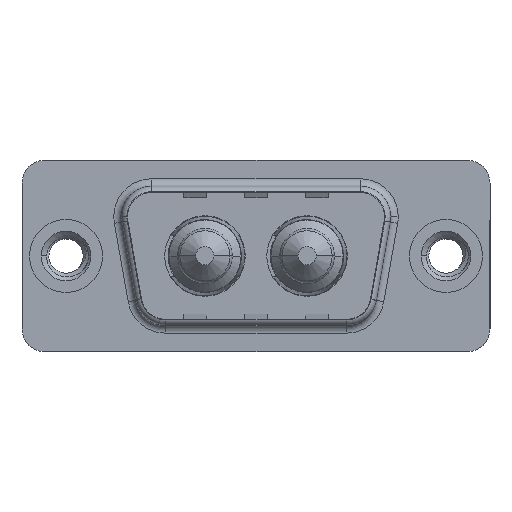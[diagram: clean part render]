
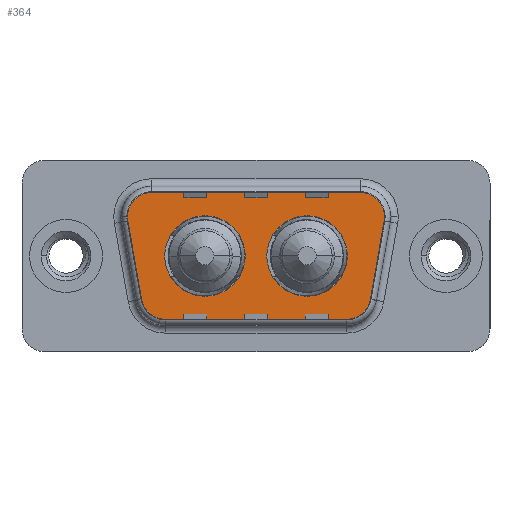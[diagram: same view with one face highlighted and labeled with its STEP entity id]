
A CAD part, top view. The second image highlights one B-rep face of the part: STEP entity #364.
In plain terms, the highlighted planar face has unit normal (0, 0, 1).
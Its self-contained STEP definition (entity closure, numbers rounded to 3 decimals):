
#38 = AXIS2_PLACEMENT_3D ( 'NONE', #1560, #8063, #2485 ) ;
#93 = CARTESIAN_POINT ( 'NONE',  ( 19.564, 2.9, 0. ) ) ;
#279 = CIRCLE ( 'NONE', #2999, 2.65 ) ;
#339 = ORIENTED_EDGE ( 'NONE', *, *, #10222, .T. ) ;
#352 = AXIS2_PLACEMENT_3D ( 'NONE', #7111, #1551, #8054 ) ;
#364 = ADVANCED_FACE ( 'NONE', ( #7872, #2904, #735 ), #11195, .T. ) ;
#393 = DIRECTION ( 'NONE',  ( 0., 0., 1. ) ) ;
#396 = AXIS2_PLACEMENT_3D ( 'NONE', #7587, #2021, #8519 ) ;
#509 = CARTESIAN_POINT ( 'NONE',  ( 15.86, 0., 0. ) ) ;
#714 = CIRCLE ( 'NONE', #3852, 2.65 ) ;
#735 = FACE_OUTER_BOUND ( 'NONE', #986, .T. ) ;
#771 = DIRECTION ( 'NONE',  ( 1., 0., 0. ) ) ;
#777 = CARTESIAN_POINT ( 'NONE',  ( 11.79, 0., 0. ) ) ;
#908 = VERTEX_POINT ( 'NONE', #11458 ) ;
#986 = EDGE_LOOP ( 'NONE', ( #3977, #2507, #9178, #2822, #2939, #3362, #339, #5074, #2088 ) ) ;
#1273 = ORIENTED_EDGE ( 'NONE', *, *, #1578, .F. ) ;
#1403 = DIRECTION ( 'NONE',  ( 1., 0., 0. ) ) ;
#1448 = DIRECTION ( 'NONE',  ( 1., 0., 0. ) ) ;
#1551 = DIRECTION ( 'NONE',  ( 0., 0., 1. ) ) ;
#1560 = CARTESIAN_POINT ( 'NONE',  ( 5.436, 2.9, 0. ) ) ;
#1578 = EDGE_CURVE ( 'NONE', #11926, #2468, #714, .T. ) ;
#1616 = CARTESIAN_POINT ( 'NONE',  ( 20.511, -3.247, 0. ) ) ;
#1685 = DIRECTION ( 'NONE',  ( -1., 0., 0. ) ) ;
#1710 = DIRECTION ( 'NONE',  ( 0., 0., 1. ) ) ;
#1712 = CARTESIAN_POINT ( 'NONE',  ( 21.564, 2.9, 0. ) ) ;
#1871 = EDGE_CURVE ( 'NONE', #2468, #11926, #279, .T. ) ;
#1943 = AXIS2_PLACEMENT_3D ( 'NONE', #509, #7012, #1448 ) ;
#1998 = CIRCLE ( 'NONE', #1943, 2.65 ) ;
#2021 = DIRECTION ( 'NONE',  ( 0., 0., 1. ) ) ;
#2088 = ORIENTED_EDGE ( 'NONE', *, *, #9169, .T. ) ;
#2161 = LINE ( 'NONE', #9250, #4331 ) ;
#2251 = VECTOR ( 'NONE', #11970, 1000. ) ;
#2264 = ORIENTED_EDGE ( 'NONE', *, *, #7090, .F. ) ;
#2468 = VERTEX_POINT ( 'NONE', #9213 ) ;
#2485 = DIRECTION ( 'NONE',  ( 1., 0., 0. ) ) ;
#2507 = ORIENTED_EDGE ( 'NONE', *, *, #4320, .T. ) ;
#2779 = EDGE_LOOP ( 'NONE', ( #2264, #5997 ) ) ;
#2822 = ORIENTED_EDGE ( 'NONE', *, *, #5196, .T. ) ;
#2904 = FACE_BOUND ( 'NONE', #9049, .T. ) ;
#2939 = ORIENTED_EDGE ( 'NONE', *, *, #6169, .T. ) ;
#2999 = AXIS2_PLACEMENT_3D ( 'NONE', #10665, #8301, #1403 ) ;
#3227 = VERTEX_POINT ( 'NONE', #1712 ) ;
#3351 = CARTESIAN_POINT ( 'NONE',  ( 18.541, -2.9, 0. ) ) ;
#3362 = ORIENTED_EDGE ( 'NONE', *, *, #9053, .T. ) ;
#3473 = EDGE_CURVE ( 'NONE', #9701, #10639, #11126, .T. ) ;
#3543 = CIRCLE ( 'NONE', #38, 2. ) ;
#3703 = CIRCLE ( 'NONE', #396, 2. ) ;
#3784 = CARTESIAN_POINT ( 'NONE',  ( 18.541, -4.9, 0. ) ) ;
#3852 = AXIS2_PLACEMENT_3D ( 'NONE', #6320, #8815, #3908 ) ;
#3908 = DIRECTION ( 'NONE',  ( 1., 0., 0. ) ) ;
#3977 = ORIENTED_EDGE ( 'NONE', *, *, #8643, .T. ) ;
#4039 = DIRECTION ( 'NONE',  ( 1., 0., 0. ) ) ;
#4287 = VECTOR ( 'NONE', #771, 1000. ) ;
#4320 = EDGE_CURVE ( 'NONE', #4610, #6914, #2161, .T. ) ;
#4331 = VECTOR ( 'NONE', #8537, 1000. ) ;
#4422 = AXIS2_PLACEMENT_3D ( 'NONE', #5977, #393, #6894 ) ;
#4610 = VERTEX_POINT ( 'NONE', #1616 ) ;
#4792 = CIRCLE ( 'NONE', #4422, 2.65 ) ;
#5074 = ORIENTED_EDGE ( 'NONE', *, *, #3473, .T. ) ;
#5196 = EDGE_CURVE ( 'NONE', #3227, #908, #9450, .T. ) ;
#5315 = LINE ( 'NONE', #11024, #2251 ) ;
#5463 = CARTESIAN_POINT ( 'NONE',  ( 5.436, 4.9, 0. ) ) ;
#5670 = VECTOR ( 'NONE', #12051, 1000. ) ;
#5899 = DIRECTION ( 'NONE',  ( 0., 0., 1. ) ) ;
#5977 = CARTESIAN_POINT ( 'NONE',  ( 15.86, 0., 0. ) ) ;
#5997 = ORIENTED_EDGE ( 'NONE', *, *, #8282, .F. ) ;
#6048 = CARTESIAN_POINT ( 'NONE',  ( 6.459, -2.9, 0. ) ) ;
#6169 = EDGE_CURVE ( 'NONE', #908, #7446, #10679, .T. ) ;
#6226 = AXIS2_PLACEMENT_3D ( 'NONE', #6048, #6653, #9906 ) ;
#6279 = AXIS2_PLACEMENT_3D ( 'NONE', #3351, #5899, #4039 ) ;
#6320 = CARTESIAN_POINT ( 'NONE',  ( 9.14, 0., 0. ) ) ;
#6476 = CARTESIAN_POINT ( 'NONE',  ( 4.489, -3.247, 0. ) ) ;
#6653 = DIRECTION ( 'NONE',  ( 0., 0., 1. ) ) ;
#6812 = CARTESIAN_POINT ( 'NONE',  ( 3.466, 2.553, 0. ) ) ;
#6894 = DIRECTION ( 'NONE',  ( 1., 0., 0. ) ) ;
#6914 = VERTEX_POINT ( 'NONE', #11344 ) ;
#7012 = DIRECTION ( 'NONE',  ( 0., 0., 1. ) ) ;
#7090 = EDGE_CURVE ( 'NONE', #11493, #10628, #4792, .T. ) ;
#7111 = CARTESIAN_POINT ( 'NONE',  ( 19.564, 2.9, 0. ) ) ;
#7435 = VERTEX_POINT ( 'NONE', #3784 ) ;
#7446 = VERTEX_POINT ( 'NONE', #10365 ) ;
#7587 = CARTESIAN_POINT ( 'NONE',  ( 18.541, -2.9, 0. ) ) ;
#7706 = CARTESIAN_POINT ( 'NONE',  ( 18.51, 0., 0. ) ) ;
#7872 = FACE_BOUND ( 'NONE', #2779, .T. ) ;
#8007 = AXIS2_PLACEMENT_3D ( 'NONE', #93, #1710, #1685 ) ;
#8054 = DIRECTION ( 'NONE',  ( -1., 0., 0. ) ) ;
#8063 = DIRECTION ( 'NONE',  ( 0., 0., 1. ) ) ;
#8282 = EDGE_CURVE ( 'NONE', #10628, #11493, #1998, .T. ) ;
#8301 = DIRECTION ( 'NONE',  ( 0., 0., 1. ) ) ;
#8519 = DIRECTION ( 'NONE',  ( 1., 0., 0. ) ) ;
#8537 = DIRECTION ( 'NONE',  ( 0.174, 0.985, 0. ) ) ;
#8643 = EDGE_CURVE ( 'NONE', #7435, #4610, #3703, .T. ) ;
#8650 = ORIENTED_EDGE ( 'NONE', *, *, #1871, .F. ) ;
#8777 = CARTESIAN_POINT ( 'NONE',  ( 13.21, 0., 0. ) ) ;
#8815 = DIRECTION ( 'NONE',  ( 0., 0., 1. ) ) ;
#9049 = EDGE_LOOP ( 'NONE', ( #1273, #8650 ) ) ;
#9053 = EDGE_CURVE ( 'NONE', #7446, #9296, #3543, .T. ) ;
#9169 = EDGE_CURVE ( 'NONE', #10639, #7435, #11816, .T. ) ;
#9178 = ORIENTED_EDGE ( 'NONE', *, *, #10163, .T. ) ;
#9213 = CARTESIAN_POINT ( 'NONE',  ( 6.49, 0., 0. ) ) ;
#9250 = CARTESIAN_POINT ( 'NONE',  ( 21.534, 2.553, 0. ) ) ;
#9296 = VERTEX_POINT ( 'NONE', #6812 ) ;
#9450 = CIRCLE ( 'NONE', #8007, 2. ) ;
#9701 = VERTEX_POINT ( 'NONE', #6476 ) ;
#9906 = DIRECTION ( 'NONE',  ( -1., 0., 0. ) ) ;
#10163 = EDGE_CURVE ( 'NONE', #6914, #3227, #11509, .T. ) ;
#10222 = EDGE_CURVE ( 'NONE', #9296, #9701, #5315, .T. ) ;
#10365 = CARTESIAN_POINT ( 'NONE',  ( 5.436, 4.9, 0. ) ) ;
#10628 = VERTEX_POINT ( 'NONE', #8777 ) ;
#10639 = VERTEX_POINT ( 'NONE', #10729 ) ;
#10665 = CARTESIAN_POINT ( 'NONE',  ( 9.14, 0., 0. ) ) ;
#10679 = LINE ( 'NONE', #5463, #5670 ) ;
#10729 = CARTESIAN_POINT ( 'NONE',  ( 6.459, -4.9, 0. ) ) ;
#11024 = CARTESIAN_POINT ( 'NONE',  ( 3.466, 2.553, 0. ) ) ;
#11101 = CARTESIAN_POINT ( 'NONE',  ( 6.459, -4.9, 0. ) ) ;
#11126 = CIRCLE ( 'NONE', #6226, 2. ) ;
#11195 = PLANE ( 'NONE',  #6279 ) ;
#11344 = CARTESIAN_POINT ( 'NONE',  ( 21.534, 2.553, 0. ) ) ;
#11458 = CARTESIAN_POINT ( 'NONE',  ( 19.564, 4.9, 0. ) ) ;
#11493 = VERTEX_POINT ( 'NONE', #7706 ) ;
#11509 = CIRCLE ( 'NONE', #352, 2. ) ;
#11816 = LINE ( 'NONE', #11101, #4287 ) ;
#11926 = VERTEX_POINT ( 'NONE', #777 ) ;
#11970 = DIRECTION ( 'NONE',  ( 0.174, -0.985, 0. ) ) ;
#12051 = DIRECTION ( 'NONE',  ( -1., 0., 0. ) ) ;
